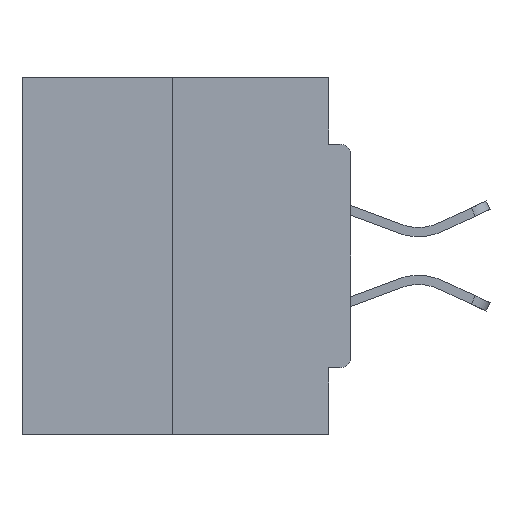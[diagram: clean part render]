
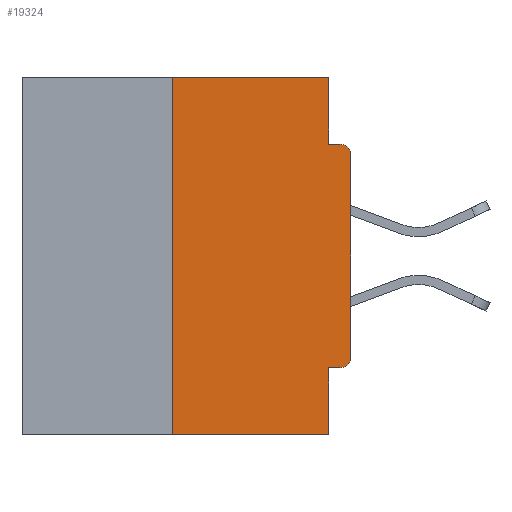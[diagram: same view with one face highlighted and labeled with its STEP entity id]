
A CAD part, left-side view. The second image highlights one B-rep face of the part: STEP entity #19324.
In plain terms, the highlighted planar face has unit normal (-1, 0, 0).
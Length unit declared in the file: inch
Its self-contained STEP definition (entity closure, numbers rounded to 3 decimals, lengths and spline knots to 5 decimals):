
#424 = ORIENTED_EDGE ( 'NONE', *, *, #30421, .F. ) ;
#772 = EDGE_CURVE ( 'NONE', #10146, #9939, #12377, .T. ) ;
#1333 = EDGE_CURVE ( 'NONE', #30357, #31703, #25198, .T. ) ;
#1350 = VERTEX_POINT ( 'NONE', #9551 ) ;
#1566 = DIRECTION ( 'NONE',  ( 0., 0., 1. ) ) ;
#2407 = VERTEX_POINT ( 'NONE', #21529 ) ;
#2599 = VERTEX_POINT ( 'NONE', #23279 ) ;
#2600 = ORIENTED_EDGE ( 'NONE', *, *, #29575, .F. ) ;
#2697 = CARTESIAN_POINT ( 'NONE',  ( 0., 0.46, 0. ) ) ;
#3132 = VECTOR ( 'NONE', #8769, 39.37008 ) ;
#3686 = ORIENTED_EDGE ( 'NONE', *, *, #3760, .T. ) ;
#3750 = CARTESIAN_POINT ( 'NONE',  ( 0., 0.46, 0. ) ) ;
#3760 = EDGE_CURVE ( 'NONE', #1350, #14196, #5318, .T. ) ;
#4082 = AXIS2_PLACEMENT_3D ( 'NONE', #16179, #28528, #8865 ) ;
#4167 = CARTESIAN_POINT ( 'NONE',  ( 0., 0., 0. ) ) ;
#4249 = CARTESIAN_POINT ( 'NONE',  ( 0., 0.031, -0.5 ) ) ;
#5014 = CARTESIAN_POINT ( 'NONE',  ( 0., 0.015, -0.4065 ) ) ;
#5318 = LINE ( 'NONE', #13179, #8450 ) ;
#6254 = ORIENTED_EDGE ( 'NONE', *, *, #1333, .F. ) ;
#6344 = EDGE_CURVE ( 'NONE', #10146, #2599, #6361, .T. ) ;
#6361 = CIRCLE ( 'NONE', #30492, 0.015 ) ;
#6649 = AXIS2_PLACEMENT_3D ( 'NONE', #2697, #9762, #20220 ) ;
#7425 = FACE_OUTER_BOUND ( 'NONE', #14916, .T. ) ;
#7520 = DIRECTION ( 'NONE',  ( -1., 0., 0. ) ) ;
#7674 = CARTESIAN_POINT ( 'NONE',  ( 0., 0.25, 0. ) ) ;
#7695 = CARTESIAN_POINT ( 'NONE',  ( 0., 0.015, -0.0935 ) ) ;
#8450 = VECTOR ( 'NONE', #25647, 39.37008 ) ;
#8769 = DIRECTION ( 'NONE',  ( 0., -1., 0. ) ) ;
#8865 = DIRECTION ( 'NONE',  ( 0., 0., -1. ) ) ;
#9551 = CARTESIAN_POINT ( 'NONE',  ( 0., 0.25, -0.5 ) ) ;
#9762 = DIRECTION ( 'NONE',  ( 1., 0., 0. ) ) ;
#9939 = VERTEX_POINT ( 'NONE', #11687 ) ;
#10043 = DIRECTION ( 'NONE',  ( 0., 0., -1. ) ) ;
#10146 = VERTEX_POINT ( 'NONE', #5014 ) ;
#10355 = EDGE_CURVE ( 'NONE', #2599, #22911, #14242, .T. ) ;
#10523 = ORIENTED_EDGE ( 'NONE', *, *, #30569, .T. ) ;
#10804 = ORIENTED_EDGE ( 'NONE', *, *, #10355, .T. ) ;
#11687 = CARTESIAN_POINT ( 'NONE',  ( 0., 0.031, -0.4065 ) ) ;
#12014 = DIRECTION ( 'NONE',  ( 0., 1., 0. ) ) ;
#12284 = CARTESIAN_POINT ( 'NONE',  ( 0., 0.25, 0. ) ) ;
#12377 = LINE ( 'NONE', #26869, #22099 ) ;
#12578 = CARTESIAN_POINT ( 'NONE',  ( 0., 0., -0.1085 ) ) ;
#13179 = CARTESIAN_POINT ( 'NONE',  ( 0., 0.46, -0.5 ) ) ;
#13451 = ORIENTED_EDGE ( 'NONE', *, *, #13701, .F. ) ;
#13608 = ORIENTED_EDGE ( 'NONE', *, *, #25935, .F. ) ;
#13701 = EDGE_CURVE ( 'NONE', #20413, #2407, #16748, .T. ) ;
#14196 = VERTEX_POINT ( 'NONE', #23439 ) ;
#14242 = LINE ( 'NONE', #4167, #18144 ) ;
#14346 = VECTOR ( 'NONE', #31633, 39.37008 ) ;
#14459 = VECTOR ( 'NONE', #25116, 39.37008 ) ;
#14916 = EDGE_LOOP ( 'NONE', ( #13451, #13608, #3686, #424, #22833, #20965, #10804, #10523, #6254, #2600 ) ) ;
#14956 = CARTESIAN_POINT ( 'NONE',  ( 0., 0.015, -0.3915 ) ) ;
#15126 = PLANE ( 'NONE',  #6649 ) ;
#15260 = LINE ( 'NONE', #7674, #14459 ) ;
#16179 = CARTESIAN_POINT ( 'NONE',  ( 0., 0.015, -0.1085 ) ) ;
#16748 = LINE ( 'NONE', #3750, #3132 ) ;
#17058 = CARTESIAN_POINT ( 'NONE',  ( 0., 0., -0.0935 ) ) ;
#17640 = CARTESIAN_POINT ( 'NONE',  ( 0., 0.031, 0. ) ) ;
#18144 = VECTOR ( 'NONE', #1566, 39.37008 ) ;
#18659 = VECTOR ( 'NONE', #20818, 39.37008 ) ;
#19324 = ADVANCED_FACE ( 'NONE', ( #7425 ), #15126, .F. ) ;
#19816 = LINE ( 'NONE', #4249, #18659 ) ;
#20220 = DIRECTION ( 'NONE',  ( 0., 0., -1. ) ) ;
#20413 = VERTEX_POINT ( 'NONE', #12284 ) ;
#20818 = DIRECTION ( 'NONE',  ( 0., 0., -1. ) ) ;
#20965 = ORIENTED_EDGE ( 'NONE', *, *, #6344, .T. ) ;
#21529 = CARTESIAN_POINT ( 'NONE',  ( 0., 0.031, 0. ) ) ;
#22099 = VECTOR ( 'NONE', #12014, 39.37008 ) ;
#22833 = ORIENTED_EDGE ( 'NONE', *, *, #772, .F. ) ;
#22911 = VERTEX_POINT ( 'NONE', #12578 ) ;
#23279 = CARTESIAN_POINT ( 'NONE',  ( 0., 0., -0.3915 ) ) ;
#23439 = CARTESIAN_POINT ( 'NONE',  ( 0., 0.031, -0.5 ) ) ;
#23786 = VECTOR ( 'NONE', #25028, 39.37008 ) ;
#24546 = LINE ( 'NONE', #17640, #23786 ) ;
#25028 = DIRECTION ( 'NONE',  ( 0., 0., -1. ) ) ;
#25116 = DIRECTION ( 'NONE',  ( 0., 0., 1. ) ) ;
#25198 = LINE ( 'NONE', #17058, #14346 ) ;
#25286 = CIRCLE ( 'NONE', #4082, 0.015 ) ;
#25647 = DIRECTION ( 'NONE',  ( 0., -1., 0. ) ) ;
#25935 = EDGE_CURVE ( 'NONE', #1350, #20413, #15260, .T. ) ;
#26019 = CARTESIAN_POINT ( 'NONE',  ( 0., 0.031, -0.0935 ) ) ;
#26869 = CARTESIAN_POINT ( 'NONE',  ( 0., 0., -0.4065 ) ) ;
#28528 = DIRECTION ( 'NONE',  ( -1., 0., 0. ) ) ;
#29575 = EDGE_CURVE ( 'NONE', #2407, #30357, #24546, .T. ) ;
#30357 = VERTEX_POINT ( 'NONE', #26019 ) ;
#30421 = EDGE_CURVE ( 'NONE', #9939, #14196, #19816, .T. ) ;
#30492 = AXIS2_PLACEMENT_3D ( 'NONE', #14956, #7520, #10043 ) ;
#30569 = EDGE_CURVE ( 'NONE', #22911, #31703, #25286, .T. ) ;
#31633 = DIRECTION ( 'NONE',  ( 0., -1., 0. ) ) ;
#31703 = VERTEX_POINT ( 'NONE', #7695 ) ;
